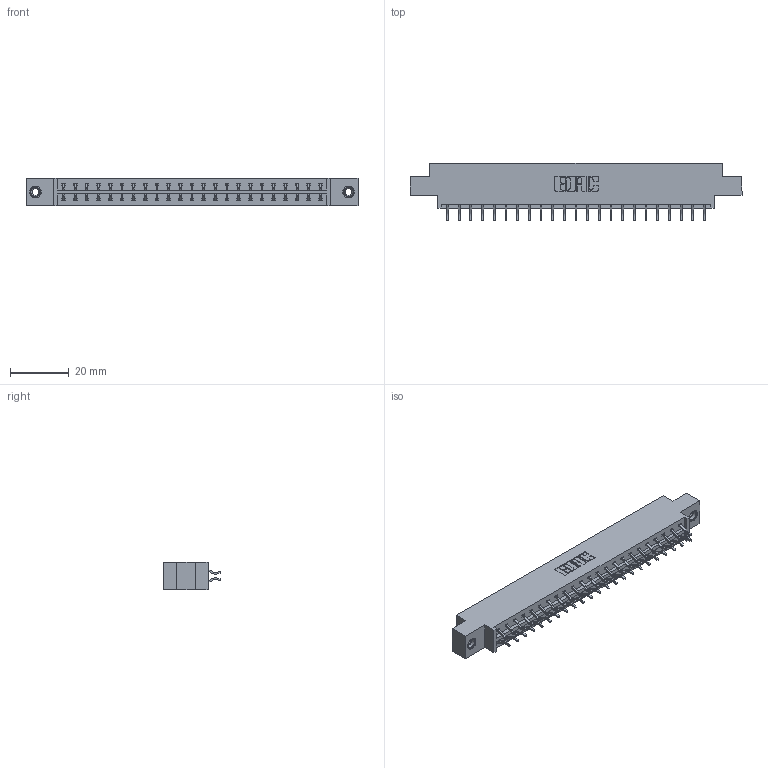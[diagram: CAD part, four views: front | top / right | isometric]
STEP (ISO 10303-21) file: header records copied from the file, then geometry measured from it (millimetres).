
FILE_DESCRIPTION (( 'STEP AP203' ), '1' );
FILE_NAME ('333-046-556-808.STEP', '2018-08-03T22:48:21', ( '' ), ( '' ), 'SwSTEP 2.0', 'SolidWorks 2016', '' );
FILE_SCHEMA (( 'CONFIG_CONTROL_DESIGN' ));
Length unit declared in the file: inch
Products named in the file (4): 333-046-556-808; 333 Part_Offset - .156 Dia - TI; 345-292-001_556 Tail; 345-250-001_345-250-003-102
Assembly tree (49 placements, depth 2):
  333-046-556-808
    333 Part_Offset - .156 Dia - TI
    345-292-001_556 Tail  x46
    345-250-001_345-250-003-102  x2
Bounding box: 112.67 x 19.57 x 9.4 mm (x, y, z)
Volume: 11089.6 mm3; surface area: 13103.7 mm2
Topology: 49 solids, 49 shells, 2846 faces, 8417 edges, 5542 vertices
Faces by surface type: plane 1946, cylinder 884, cone 12, torus 4
Entity records: 18792 total; most frequent: CARTESIAN_POINT 3137, ORIENTED_EDGE 3054, DIRECTION 2733, EDGE_CURVE 1527, VECTOR 1371, LINE 1371, VERTEX_POINT 1012, AXIS2_PLACEMENT_3D 681
